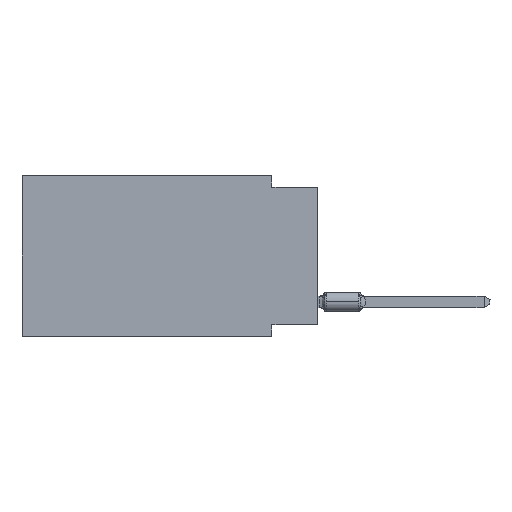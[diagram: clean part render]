
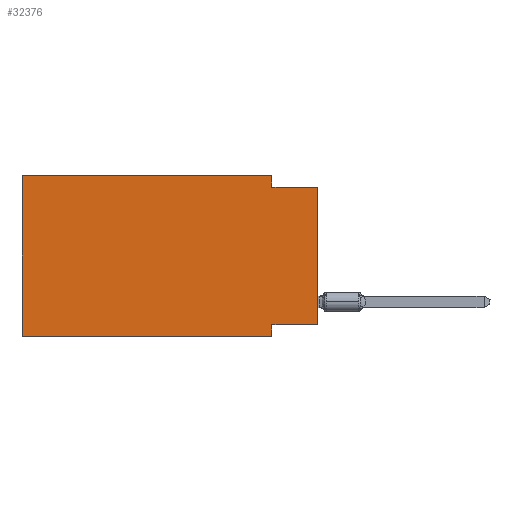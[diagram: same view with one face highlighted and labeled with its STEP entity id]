
A CAD part, left-side view. The second image highlights one B-rep face of the part: STEP entity #32376.
In plain terms, the highlighted planar face has unit normal (-1, 0, 0).
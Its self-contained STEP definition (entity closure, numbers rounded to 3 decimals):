
#5 = VERTEX_POINT ( 'NONE', #3605 ) ;
#760 = CARTESIAN_POINT ( 'NONE',  ( 0., 0., -0.635 ) ) ;
#912 = DIRECTION ( 'NONE',  ( 0., -1., 0. ) ) ;
#1054 = CARTESIAN_POINT ( 'NONE',  ( 0., 16.383, 0. ) ) ;
#1278 = CARTESIAN_POINT ( 'NONE',  ( 0., 0., 0. ) ) ;
#1843 = DIRECTION ( 'NONE',  ( 0., -1., 0. ) ) ;
#2605 = DIRECTION ( 'NONE',  ( 0., 0., -1. ) ) ;
#3605 = CARTESIAN_POINT ( 'NONE',  ( 0., 2.54, -0.635 ) ) ;
#3983 = EDGE_CURVE ( 'NONE', #19415, #9744, #34551, .T. ) ;
#4240 = VECTOR ( 'NONE', #16279, 1000. ) ;
#4295 = CARTESIAN_POINT ( 'NONE',  ( 0., 16.383, 0. ) ) ;
#4860 = LINE ( 'NONE', #15504, #32744 ) ;
#5272 = LINE ( 'NONE', #29362, #4240 ) ;
#7035 = EDGE_CURVE ( 'NONE', #29524, #9744, #5272, .T. ) ;
#8107 = EDGE_CURVE ( 'NONE', #32694, #29524, #32779, .T. ) ;
#8340 = CARTESIAN_POINT ( 'NONE',  ( 0., 16.383, 0. ) ) ;
#8676 = AXIS2_PLACEMENT_3D ( 'NONE', #21453, #13072, #2605 ) ;
#9095 = CARTESIAN_POINT ( 'NONE',  ( 0., 2.54, 0. ) ) ;
#9511 = VECTOR ( 'NONE', #23311, 1000. ) ;
#9563 = CARTESIAN_POINT ( 'NONE',  ( 0., 0., -8.255 ) ) ;
#9744 = VERTEX_POINT ( 'NONE', #23025 ) ;
#9937 = EDGE_CURVE ( 'NONE', #5, #33050, #4860, .T. ) ;
#10229 = EDGE_CURVE ( 'NONE', #27016, #22241, #33970, .T. ) ;
#12853 = EDGE_CURVE ( 'NONE', #22241, #5, #17918, .T. ) ;
#12887 = VECTOR ( 'NONE', #18663, 1000. ) ;
#12920 = CARTESIAN_POINT ( 'NONE',  ( 0., 16.383, -8.89 ) ) ;
#13072 = DIRECTION ( 'NONE',  ( 1., 0., 0. ) ) ;
#13778 = ORIENTED_EDGE ( 'NONE', *, *, #3983, .T. ) ;
#15282 = CARTESIAN_POINT ( 'NONE',  ( 0., 2.54, 0. ) ) ;
#15504 = CARTESIAN_POINT ( 'NONE',  ( 0., 0., -0.635 ) ) ;
#15585 = VECTOR ( 'NONE', #27189, 1000. ) ;
#15925 = EDGE_CURVE ( 'NONE', #19415, #27016, #34529, .T. ) ;
#16279 = DIRECTION ( 'NONE',  ( 0., 0., -1. ) ) ;
#16387 = CARTESIAN_POINT ( 'NONE',  ( 0., 0., -8.255 ) ) ;
#17918 = LINE ( 'NONE', #15282, #9511 ) ;
#18663 = DIRECTION ( 'NONE',  ( 0., -1., 0. ) ) ;
#18861 = CARTESIAN_POINT ( 'NONE',  ( 0., 2.54, -8.255 ) ) ;
#19415 = VERTEX_POINT ( 'NONE', #23915 ) ;
#19429 = ORIENTED_EDGE ( 'NONE', *, *, #34255, .T. ) ;
#21453 = CARTESIAN_POINT ( 'NONE',  ( 0., 16.383, 0. ) ) ;
#21695 = ORIENTED_EDGE ( 'NONE', *, *, #7035, .F. ) ;
#21965 = ORIENTED_EDGE ( 'NONE', *, *, #12853, .F. ) ;
#22241 = VERTEX_POINT ( 'NONE', #9095 ) ;
#22829 = ORIENTED_EDGE ( 'NONE', *, *, #9937, .F. ) ;
#23025 = CARTESIAN_POINT ( 'NONE',  ( 0., 2.54, -8.89 ) ) ;
#23311 = DIRECTION ( 'NONE',  ( 0., 0., -1. ) ) ;
#23915 = CARTESIAN_POINT ( 'NONE',  ( 0., 16.383, -8.89 ) ) ;
#25197 = LINE ( 'NONE', #1278, #31662 ) ;
#25773 = ORIENTED_EDGE ( 'NONE', *, *, #8107, .F. ) ;
#26163 = PLANE ( 'NONE',  #8676 ) ;
#26497 = ORIENTED_EDGE ( 'NONE', *, *, #10229, .F. ) ;
#27016 = VERTEX_POINT ( 'NONE', #1054 ) ;
#27189 = DIRECTION ( 'NONE',  ( 0., 1., 0. ) ) ;
#27462 = DIRECTION ( 'NONE',  ( 0., 0., 1. ) ) ;
#28959 = FACE_OUTER_BOUND ( 'NONE', #33045, .T. ) ;
#29108 = DIRECTION ( 'NONE',  ( 0., 0., 1. ) ) ;
#29362 = CARTESIAN_POINT ( 'NONE',  ( 0., 2.54, -8.89 ) ) ;
#29524 = VERTEX_POINT ( 'NONE', #18861 ) ;
#31632 = VECTOR ( 'NONE', #1843, 1000. ) ;
#31662 = VECTOR ( 'NONE', #27462, 1000. ) ;
#31817 = VECTOR ( 'NONE', #29108, 1000. ) ;
#32376 = ADVANCED_FACE ( 'NONE', ( #28959 ), #26163, .F. ) ;
#32694 = VERTEX_POINT ( 'NONE', #9563 ) ;
#32744 = VECTOR ( 'NONE', #912, 1000. ) ;
#32779 = LINE ( 'NONE', #16387, #15585 ) ;
#33045 = EDGE_LOOP ( 'NONE', ( #19429, #22829, #21965, #26497, #33897, #13778, #21695, #25773 ) ) ;
#33050 = VERTEX_POINT ( 'NONE', #760 ) ;
#33897 = ORIENTED_EDGE ( 'NONE', *, *, #15925, .F. ) ;
#33970 = LINE ( 'NONE', #4295, #31632 ) ;
#34255 = EDGE_CURVE ( 'NONE', #32694, #33050, #25197, .T. ) ;
#34529 = LINE ( 'NONE', #8340, #31817 ) ;
#34551 = LINE ( 'NONE', #12920, #12887 ) ;
